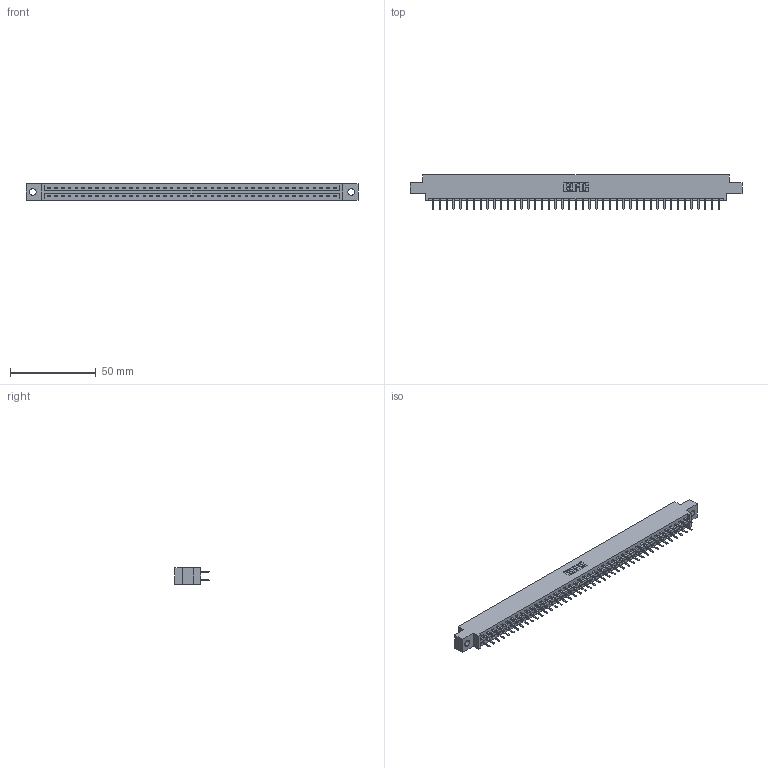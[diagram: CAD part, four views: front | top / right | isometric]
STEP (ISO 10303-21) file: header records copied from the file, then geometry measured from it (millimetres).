
FILE_DESCRIPTION (( 'STEP AP203' ), '1' );
FILE_NAME ('337-086-520-804.STEP', '2019-10-15T18:36:03', ( '' ), ( '' ), 'SwSTEP 2.0', 'SolidWorks 2016', '' );
FILE_SCHEMA (( 'CONFIG_CONTROL_DESIGN' ));
Length unit declared in the file: inch
Products named in the file (3): 345-292-001_345-293-120; 337-086-520-804; 337 Part_0.170 Offset - 0.156 Dia-TH
Assembly tree (87 placements, depth 2):
  337-086-520-804
    337 Part_0.170 Offset - 0.156 Dia-TH
    345-292-001_345-293-120  x86
Bounding box: 193.4 x 20.02 x 9.4 mm (x, y, z)
Volume: 20151.7 mm3; surface area: 22588.7 mm2
Topology: 87 solids, 87 shells, 5106 faces, 14857 edges, 9674 vertices
Faces by surface type: plane 3514, cylinder 1592
Entity records: 33459 total; most frequent: CARTESIAN_POINT 5650, ORIENTED_EDGE 5574, DIRECTION 4791, EDGE_CURVE 2787, VECTOR 2655, LINE 2655, VERTEX_POINT 1854, AXIS2_PLACEMENT_3D 1068
